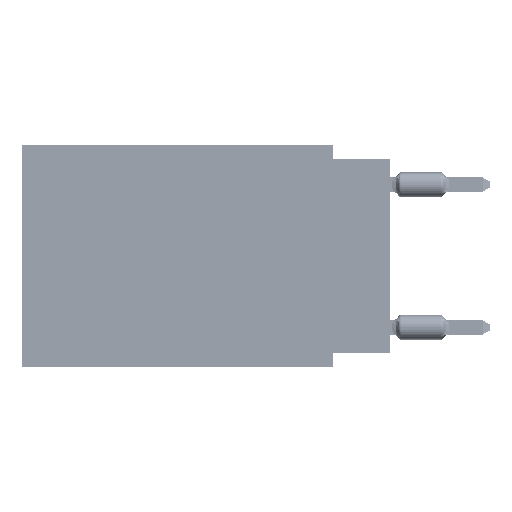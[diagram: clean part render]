
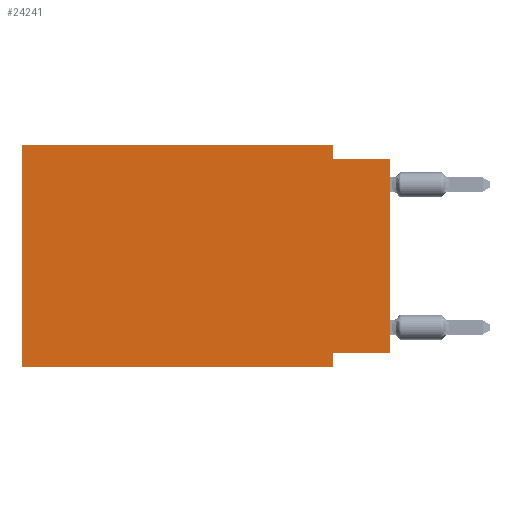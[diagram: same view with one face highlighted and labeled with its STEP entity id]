
A CAD part, left-side view. The second image highlights one B-rep face of the part: STEP entity #24241.
In plain terms, the highlighted planar face has unit normal (-1, 0, 0).
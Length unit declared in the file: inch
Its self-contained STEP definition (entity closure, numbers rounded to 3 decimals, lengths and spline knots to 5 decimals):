
#671 = CARTESIAN_POINT ( 'NONE',  ( 0., 0.1, -0.365 ) ) ;
#1848 = DIRECTION ( 'NONE',  ( 0., 0., -1. ) ) ;
#4949 = LINE ( 'NONE', #53476, #54322 ) ;
#5491 = DIRECTION ( 'NONE',  ( 0., 0., -1. ) ) ;
#5830 = DIRECTION ( 'NONE',  ( 0., -1., 0. ) ) ;
#6369 = CARTESIAN_POINT ( 'NONE',  ( 0., 0., 0. ) ) ;
#6537 = CARTESIAN_POINT ( 'NONE',  ( 0., 0., -0.365 ) ) ;
#11521 = LINE ( 'NONE', #6537, #30330 ) ;
#14619 = EDGE_CURVE ( 'NONE', #85424, #69004, #60532, .T. ) ;
#16768 = ORIENTED_EDGE ( 'NONE', *, *, #72321, .F. ) ;
#18193 = EDGE_CURVE ( 'NONE', #84102, #23349, #67956, .T. ) ;
#19813 = VECTOR ( 'NONE', #60511, 39.37008 ) ;
#20029 = CARTESIAN_POINT ( 'NONE',  ( 0., 0.645, 0. ) ) ;
#20214 = ORIENTED_EDGE ( 'NONE', *, *, #56116, .F. ) ;
#20816 = VECTOR ( 'NONE', #47041, 39.37008 ) ;
#23349 = VERTEX_POINT ( 'NONE', #43177 ) ;
#23818 = CARTESIAN_POINT ( 'NONE',  ( 0., 0.645, 0. ) ) ;
#24241 = ADVANCED_FACE ( 'NONE', ( #33348 ), #47738, .F. ) ;
#25298 = CARTESIAN_POINT ( 'NONE',  ( 0., 0.1, -0.025 ) ) ;
#27476 = CARTESIAN_POINT ( 'NONE',  ( 0., 0.1, 0. ) ) ;
#27934 = ORIENTED_EDGE ( 'NONE', *, *, #41343, .F. ) ;
#30330 = VECTOR ( 'NONE', #46571, 39.37008 ) ;
#33044 = CARTESIAN_POINT ( 'NONE',  ( 0., 0., -0.365 ) ) ;
#33348 = FACE_OUTER_BOUND ( 'NONE', #57237, .T. ) ;
#33776 = DIRECTION ( 'NONE',  ( 1., 0., 0. ) ) ;
#33949 = LINE ( 'NONE', #20029, #52853 ) ;
#34280 = ORIENTED_EDGE ( 'NONE', *, *, #18193, .T. ) ;
#35656 = VECTOR ( 'NONE', #38685, 39.37008 ) ;
#38685 = DIRECTION ( 'NONE',  ( 0., 0., 1. ) ) ;
#39138 = VECTOR ( 'NONE', #1848, 39.37008 ) ;
#41343 = EDGE_CURVE ( 'NONE', #62596, #63897, #58026, .T. ) ;
#41453 = EDGE_CURVE ( 'NONE', #62596, #69004, #4949, .T. ) ;
#41579 = CARTESIAN_POINT ( 'NONE',  ( 0., 0.645, -0.39 ) ) ;
#43177 = CARTESIAN_POINT ( 'NONE',  ( 0., 0., -0.025 ) ) ;
#43802 = ORIENTED_EDGE ( 'NONE', *, *, #14619, .F. ) ;
#46146 = CARTESIAN_POINT ( 'NONE',  ( 0., 0.1, -0.39 ) ) ;
#46571 = DIRECTION ( 'NONE',  ( 0., 1., 0. ) ) ;
#47041 = DIRECTION ( 'NONE',  ( 0., 0., -1. ) ) ;
#47738 = PLANE ( 'NONE',  #85820 ) ;
#49057 = LINE ( 'NONE', #27476, #39138 ) ;
#51792 = CARTESIAN_POINT ( 'NONE',  ( 0., 0.1, 0. ) ) ;
#52853 = VECTOR ( 'NONE', #74856, 39.37008 ) ;
#53476 = CARTESIAN_POINT ( 'NONE',  ( 0., 0.645, -0.39 ) ) ;
#54322 = VECTOR ( 'NONE', #5830, 39.37008 ) ;
#56116 = EDGE_CURVE ( 'NONE', #84102, #85424, #11521, .T. ) ;
#57237 = EDGE_LOOP ( 'NONE', ( #34280, #75939, #60713, #16768, #27934, #80714, #43802, #20214 ) ) ;
#58026 = LINE ( 'NONE', #23818, #35656 ) ;
#59969 = VERTEX_POINT ( 'NONE', #51792 ) ;
#60511 = DIRECTION ( 'NONE',  ( 0., -1., 0. ) ) ;
#60532 = LINE ( 'NONE', #81636, #20816 ) ;
#60713 = ORIENTED_EDGE ( 'NONE', *, *, #77998, .F. ) ;
#60953 = LINE ( 'NONE', #73538, #19813 ) ;
#62596 = VERTEX_POINT ( 'NONE', #41579 ) ;
#63897 = VERTEX_POINT ( 'NONE', #70772 ) ;
#66524 = VERTEX_POINT ( 'NONE', #25298 ) ;
#67956 = LINE ( 'NONE', #6369, #82745 ) ;
#67959 = CARTESIAN_POINT ( 'NONE',  ( 0., 0.645, 0. ) ) ;
#69004 = VERTEX_POINT ( 'NONE', #46146 ) ;
#70772 = CARTESIAN_POINT ( 'NONE',  ( 0., 0.645, 0. ) ) ;
#72279 = EDGE_CURVE ( 'NONE', #66524, #23349, #60953, .T. ) ;
#72321 = EDGE_CURVE ( 'NONE', #63897, #59969, #33949, .T. ) ;
#73538 = CARTESIAN_POINT ( 'NONE',  ( 0., 0., -0.025 ) ) ;
#74856 = DIRECTION ( 'NONE',  ( 0., -1., 0. ) ) ;
#75939 = ORIENTED_EDGE ( 'NONE', *, *, #72279, .F. ) ;
#77998 = EDGE_CURVE ( 'NONE', #59969, #66524, #49057, .T. ) ;
#80714 = ORIENTED_EDGE ( 'NONE', *, *, #41453, .T. ) ;
#81435 = DIRECTION ( 'NONE',  ( 0., 0., 1. ) ) ;
#81636 = CARTESIAN_POINT ( 'NONE',  ( 0., 0.1, -0.39 ) ) ;
#82745 = VECTOR ( 'NONE', #81435, 39.37008 ) ;
#84102 = VERTEX_POINT ( 'NONE', #33044 ) ;
#85424 = VERTEX_POINT ( 'NONE', #671 ) ;
#85820 = AXIS2_PLACEMENT_3D ( 'NONE', #67959, #33776, #5491 ) ;
